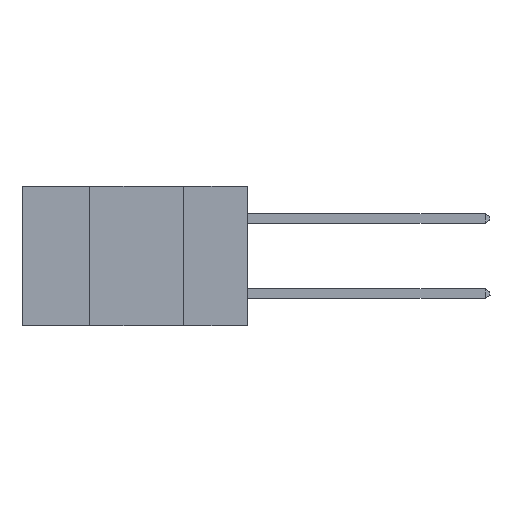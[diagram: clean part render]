
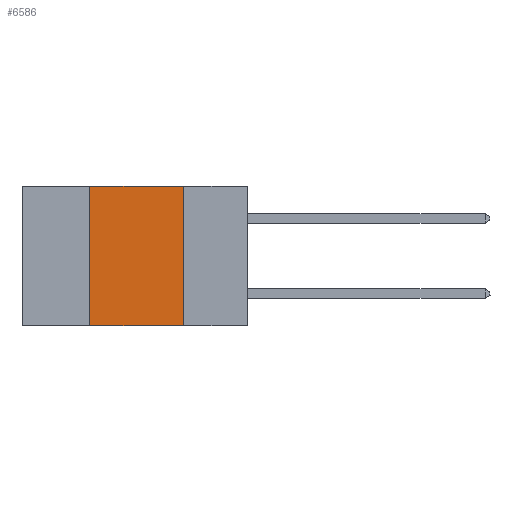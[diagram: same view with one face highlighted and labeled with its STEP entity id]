
A CAD part, left-side view. The second image highlights one B-rep face of the part: STEP entity #6586.
In plain terms, the highlighted planar face has unit normal (-1, 0, 0).
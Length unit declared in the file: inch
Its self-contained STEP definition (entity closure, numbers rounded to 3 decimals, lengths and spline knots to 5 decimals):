
#2155 = CARTESIAN_POINT ( 'NONE',  ( 0., 0.6, -0.37 ) ) ;
#3000 = CARTESIAN_POINT ( 'NONE',  ( 0., 0.17, 0. ) ) ;
#4508 = DIRECTION ( 'NONE',  ( 0., 0., 1. ) ) ;
#5254 = AXIS2_PLACEMENT_3D ( 'NONE', #22264, #22355, #6830 ) ;
#5459 = VECTOR ( 'NONE', #19884, 39.37008 ) ;
#5591 = FACE_OUTER_BOUND ( 'NONE', #22659, .T. ) ;
#6586 = ADVANCED_FACE ( 'NONE', ( #5591 ), #20244, .F. ) ;
#6830 = DIRECTION ( 'NONE',  ( 0., 0., -1. ) ) ;
#7153 = LINE ( 'NONE', #2155, #18491 ) ;
#7228 = VERTEX_POINT ( 'NONE', #14708 ) ;
#8513 = LINE ( 'NONE', #3000, #21128 ) ;
#8605 = CARTESIAN_POINT ( 'NONE',  ( 0., 0.42, -0.37 ) ) ;
#9505 = LINE ( 'NONE', #14554, #23113 ) ;
#9852 = LINE ( 'NONE', #17773, #5459 ) ;
#11582 = EDGE_CURVE ( 'NONE', #13778, #24288, #9505, .T. ) ;
#13460 = ORIENTED_EDGE ( 'NONE', *, *, #19125, .F. ) ;
#13603 = CARTESIAN_POINT ( 'NONE',  ( 0., 0.42, 0. ) ) ;
#13778 = VERTEX_POINT ( 'NONE', #8605 ) ;
#13992 = DIRECTION ( 'NONE',  ( 0., -1., 0. ) ) ;
#14554 = CARTESIAN_POINT ( 'NONE',  ( 0., 0.42, 0. ) ) ;
#14708 = CARTESIAN_POINT ( 'NONE',  ( 0., 0.17, 0. ) ) ;
#15264 = EDGE_CURVE ( 'NONE', #13778, #22365, #7153, .T. ) ;
#15803 = ORIENTED_EDGE ( 'NONE', *, *, #25087, .F. ) ;
#16447 = ORIENTED_EDGE ( 'NONE', *, *, #11582, .F. ) ;
#17773 = CARTESIAN_POINT ( 'NONE',  ( 0., 0.6, 0. ) ) ;
#18491 = VECTOR ( 'NONE', #13992, 39.37008 ) ;
#19125 = EDGE_CURVE ( 'NONE', #7228, #22365, #8513, .T. ) ;
#19884 = DIRECTION ( 'NONE',  ( 0., -1., 0. ) ) ;
#20244 = PLANE ( 'NONE',  #5254 ) ;
#20839 = ORIENTED_EDGE ( 'NONE', *, *, #15264, .T. ) ;
#21128 = VECTOR ( 'NONE', #25128, 39.37008 ) ;
#21824 = CARTESIAN_POINT ( 'NONE',  ( 0., 0.17, -0.37 ) ) ;
#22264 = CARTESIAN_POINT ( 'NONE',  ( 0., 0.6, 0. ) ) ;
#22355 = DIRECTION ( 'NONE',  ( 1., 0., 0. ) ) ;
#22365 = VERTEX_POINT ( 'NONE', #21824 ) ;
#22659 = EDGE_LOOP ( 'NONE', ( #13460, #15803, #16447, #20839 ) ) ;
#23113 = VECTOR ( 'NONE', #4508, 39.37008 ) ;
#24288 = VERTEX_POINT ( 'NONE', #13603 ) ;
#25087 = EDGE_CURVE ( 'NONE', #24288, #7228, #9852, .T. ) ;
#25128 = DIRECTION ( 'NONE',  ( 0., 0., -1. ) ) ;
